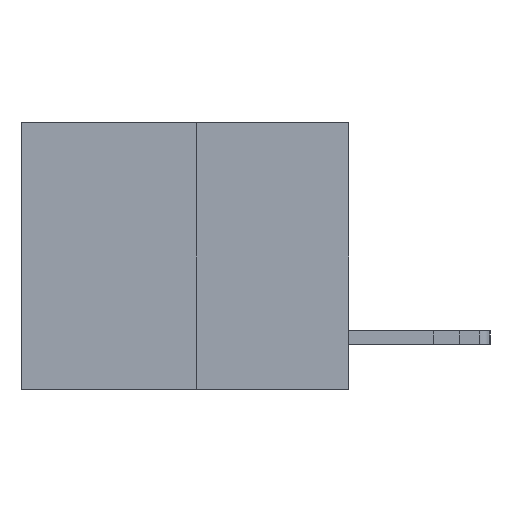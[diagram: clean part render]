
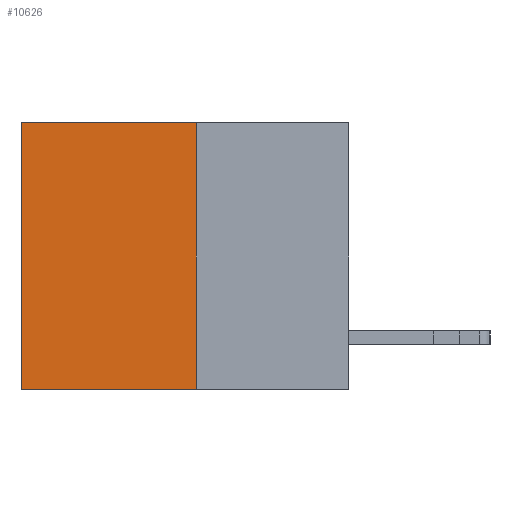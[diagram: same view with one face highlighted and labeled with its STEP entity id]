
A CAD part, left-side view. The second image highlights one B-rep face of the part: STEP entity #10626.
In plain terms, the highlighted planar face has unit normal (-1, 0, 0).
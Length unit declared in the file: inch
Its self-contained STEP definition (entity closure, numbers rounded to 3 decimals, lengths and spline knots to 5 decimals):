
#2456 = VERTEX_POINT ( 'NONE', #19880 ) ;
#2806 = VECTOR ( 'NONE', #3487, 39.37008 ) ;
#2876 = CARTESIAN_POINT ( 'NONE',  ( 0.3165, 0.6, -0.49 ) ) ;
#3487 = DIRECTION ( 'NONE',  ( 0., 1., 0. ) ) ;
#3515 = EDGE_CURVE ( 'NONE', #16474, #2456, #4249, .T. ) ;
#3570 = CARTESIAN_POINT ( 'NONE',  ( 0.3165, 0.28, 0. ) ) ;
#3944 = CARTESIAN_POINT ( 'NONE',  ( 0.3165, 0.28, -0.49 ) ) ;
#4070 = ORIENTED_EDGE ( 'NONE', *, *, #12573, .T. ) ;
#4249 = LINE ( 'NONE', #2876, #16821 ) ;
#4776 = ORIENTED_EDGE ( 'NONE', *, *, #5546, .F. ) ;
#5151 = ORIENTED_EDGE ( 'NONE', *, *, #3515, .T. ) ;
#5546 = EDGE_CURVE ( 'NONE', #18634, #2456, #15828, .T. ) ;
#6732 = PLANE ( 'NONE',  #25959 ) ;
#7004 = DIRECTION ( 'NONE',  ( 1., 0., 0. ) ) ;
#8807 = EDGE_CURVE ( 'NONE', #21048, #18634, #16320, .T. ) ;
#9138 = VECTOR ( 'NONE', #21539, 39.37008 ) ;
#10626 = ADVANCED_FACE ( 'NONE', ( #13933 ), #6732, .F. ) ;
#11056 = DIRECTION ( 'NONE',  ( 0., 0., -1. ) ) ;
#12573 = EDGE_CURVE ( 'NONE', #21048, #16474, #18186, .T. ) ;
#13933 = FACE_OUTER_BOUND ( 'NONE', #25370, .T. ) ;
#14321 = DIRECTION ( 'NONE',  ( 0., 1., 0. ) ) ;
#15028 = ORIENTED_EDGE ( 'NONE', *, *, #8807, .F. ) ;
#15179 = CARTESIAN_POINT ( 'NONE',  ( 0.3165, 0.6, 0. ) ) ;
#15828 = LINE ( 'NONE', #3944, #23734 ) ;
#16320 = LINE ( 'NONE', #23629, #9138 ) ;
#16474 = VERTEX_POINT ( 'NONE', #15179 ) ;
#16821 = VECTOR ( 'NONE', #24928, 39.37008 ) ;
#16995 = CARTESIAN_POINT ( 'NONE',  ( 0.3165, 0.28, -0.49 ) ) ;
#18186 = LINE ( 'NONE', #3570, #2806 ) ;
#18634 = VERTEX_POINT ( 'NONE', #16995 ) ;
#19001 = CARTESIAN_POINT ( 'NONE',  ( 0.3165, 0.28, -0.49 ) ) ;
#19880 = CARTESIAN_POINT ( 'NONE',  ( 0.3165, 0.6, -0.49 ) ) ;
#21048 = VERTEX_POINT ( 'NONE', #23265 ) ;
#21539 = DIRECTION ( 'NONE',  ( 0., 0., -1. ) ) ;
#23265 = CARTESIAN_POINT ( 'NONE',  ( 0.3165, 0.28, 0. ) ) ;
#23629 = CARTESIAN_POINT ( 'NONE',  ( 0.3165, 0.28, -0.49 ) ) ;
#23734 = VECTOR ( 'NONE', #14321, 39.37008 ) ;
#24928 = DIRECTION ( 'NONE',  ( 0., 0., -1. ) ) ;
#25370 = EDGE_LOOP ( 'NONE', ( #5151, #4776, #15028, #4070 ) ) ;
#25959 = AXIS2_PLACEMENT_3D ( 'NONE', #19001, #7004, #11056 ) ;
